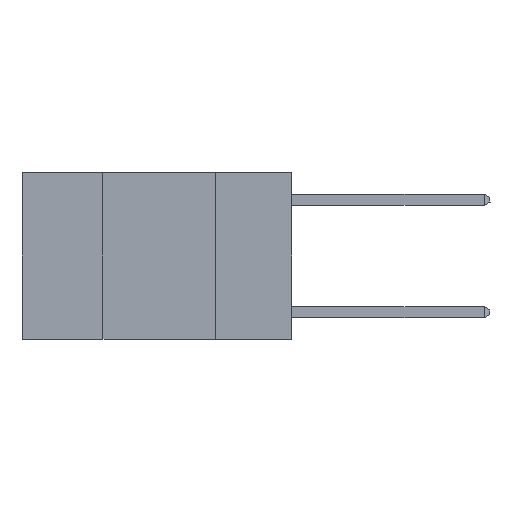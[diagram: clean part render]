
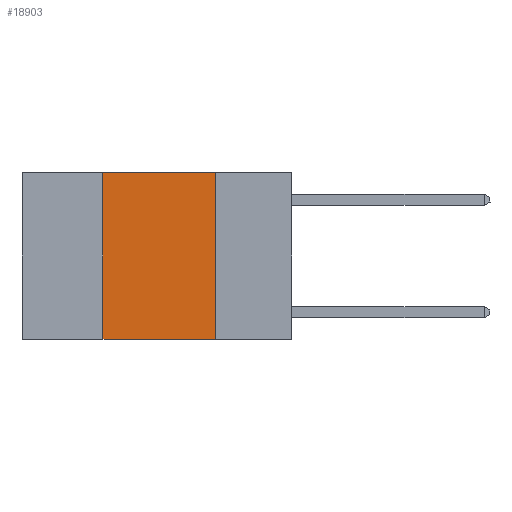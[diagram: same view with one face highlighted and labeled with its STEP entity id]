
A CAD part, left-side view. The second image highlights one B-rep face of the part: STEP entity #18903.
In plain terms, the highlighted planar face has unit normal (-1, 0, 0).
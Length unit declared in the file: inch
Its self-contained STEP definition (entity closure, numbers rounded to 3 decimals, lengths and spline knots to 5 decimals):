
#15 = LINE ( 'NONE', #1236, #5692 ) ;
#151 = CARTESIAN_POINT ( 'NONE',  ( 0., 0.42, 0. ) ) ;
#1236 = CARTESIAN_POINT ( 'NONE',  ( 0., 0.6, -0.37 ) ) ;
#1924 = LINE ( 'NONE', #24348, #7625 ) ;
#3681 = DIRECTION ( 'NONE',  ( 0., -1., 0. ) ) ;
#4144 = CARTESIAN_POINT ( 'NONE',  ( 0., 0.6, 0. ) ) ;
#4685 = ORIENTED_EDGE ( 'NONE', *, *, #7872, .F. ) ;
#5659 = FACE_OUTER_BOUND ( 'NONE', #20862, .T. ) ;
#5692 = VECTOR ( 'NONE', #3681, 39.37008 ) ;
#6300 = EDGE_CURVE ( 'NONE', #28305, #11460, #15234, .T. ) ;
#7236 = EDGE_CURVE ( 'NONE', #21895, #28305, #1924, .T. ) ;
#7625 = VECTOR ( 'NONE', #26818, 39.37008 ) ;
#7872 = EDGE_CURVE ( 'NONE', #11460, #15270, #9462, .T. ) ;
#8699 = VECTOR ( 'NONE', #29415, 39.37008 ) ;
#9462 = LINE ( 'NONE', #12452, #8699 ) ;
#10860 = DIRECTION ( 'NONE',  ( 1., 0., 0. ) ) ;
#11460 = VERTEX_POINT ( 'NONE', #27328 ) ;
#12452 = CARTESIAN_POINT ( 'NONE',  ( 0., 0.17, 0. ) ) ;
#13910 = AXIS2_PLACEMENT_3D ( 'NONE', #25397, #10860, #27829 ) ;
#14344 = ORIENTED_EDGE ( 'NONE', *, *, #31215, .T. ) ;
#15234 = LINE ( 'NONE', #4144, #28115 ) ;
#15270 = VERTEX_POINT ( 'NONE', #23058 ) ;
#15490 = CARTESIAN_POINT ( 'NONE',  ( 0., 0.42, -0.37 ) ) ;
#17015 = ORIENTED_EDGE ( 'NONE', *, *, #6300, .F. ) ;
#18903 = ADVANCED_FACE ( 'NONE', ( #5659 ), #30159, .F. ) ;
#19239 = ORIENTED_EDGE ( 'NONE', *, *, #7236, .F. ) ;
#20862 = EDGE_LOOP ( 'NONE', ( #4685, #17015, #19239, #14344 ) ) ;
#21135 = DIRECTION ( 'NONE',  ( 0., -1., 0. ) ) ;
#21895 = VERTEX_POINT ( 'NONE', #15490 ) ;
#23058 = CARTESIAN_POINT ( 'NONE',  ( 0., 0.17, -0.37 ) ) ;
#24348 = CARTESIAN_POINT ( 'NONE',  ( 0., 0.42, 0. ) ) ;
#25397 = CARTESIAN_POINT ( 'NONE',  ( 0., 0.6, 0. ) ) ;
#26818 = DIRECTION ( 'NONE',  ( 0., 0., 1. ) ) ;
#27328 = CARTESIAN_POINT ( 'NONE',  ( 0., 0.17, 0. ) ) ;
#27829 = DIRECTION ( 'NONE',  ( 0., 0., -1. ) ) ;
#28115 = VECTOR ( 'NONE', #21135, 39.37008 ) ;
#28305 = VERTEX_POINT ( 'NONE', #151 ) ;
#29415 = DIRECTION ( 'NONE',  ( 0., 0., -1. ) ) ;
#30159 = PLANE ( 'NONE',  #13910 ) ;
#31215 = EDGE_CURVE ( 'NONE', #21895, #15270, #15, .T. ) ;
